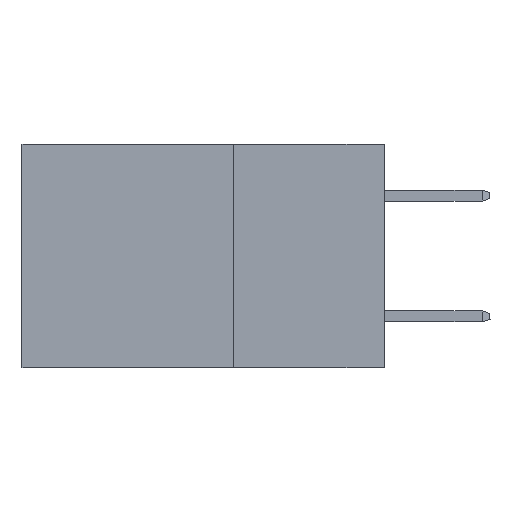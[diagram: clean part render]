
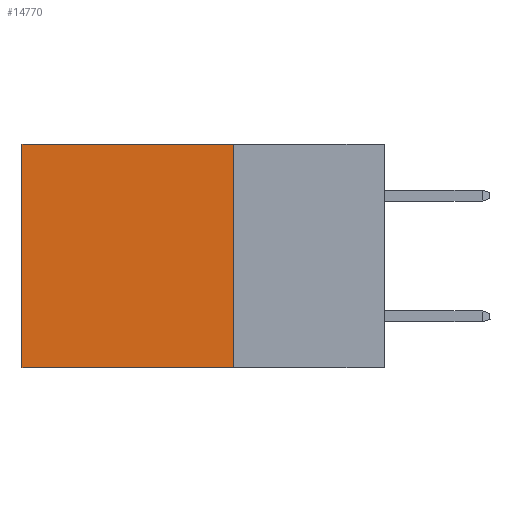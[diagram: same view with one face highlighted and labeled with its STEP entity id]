
A CAD part, left-side view. The second image highlights one B-rep face of the part: STEP entity #14770.
In plain terms, the highlighted planar face has unit normal (-1, 0, 0).
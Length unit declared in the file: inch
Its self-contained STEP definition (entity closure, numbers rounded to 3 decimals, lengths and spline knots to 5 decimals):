
#502 = CARTESIAN_POINT ( 'NONE',  ( 0.2615, 0.25, 0. ) ) ;
#1231 = ORIENTED_EDGE ( 'NONE', *, *, #18965, .T. ) ;
#3579 = EDGE_CURVE ( 'NONE', #19767, #16355, #6559, .T. ) ;
#3671 = DIRECTION ( 'NONE',  ( 0., 1., 0. ) ) ;
#4779 = VECTOR ( 'NONE', #6517, 39.37008 ) ;
#4913 = CARTESIAN_POINT ( 'NONE',  ( 0.2615, 0.25, -0.37 ) ) ;
#4959 = EDGE_CURVE ( 'NONE', #5180, #19767, #13064, .T. ) ;
#5180 = VERTEX_POINT ( 'NONE', #5378 ) ;
#5378 = CARTESIAN_POINT ( 'NONE',  ( 0.2615, 0.25, 0. ) ) ;
#5915 = CARTESIAN_POINT ( 'NONE',  ( 0.2615, 0.25, -0.37 ) ) ;
#5941 = LINE ( 'NONE', #502, #9126 ) ;
#6517 = DIRECTION ( 'NONE',  ( 0., 0., -1. ) ) ;
#6559 = LINE ( 'NONE', #12839, #9701 ) ;
#6846 = CARTESIAN_POINT ( 'NONE',  ( 0.2615, 0.6, -0.37 ) ) ;
#6908 = PLANE ( 'NONE',  #18008 ) ;
#8176 = CARTESIAN_POINT ( 'NONE',  ( 0.2615, 0.6, 0. ) ) ;
#8489 = DIRECTION ( 'NONE',  ( 0., 0., -1. ) ) ;
#9126 = VECTOR ( 'NONE', #3671, 39.37008 ) ;
#9701 = VECTOR ( 'NONE', #13713, 39.37008 ) ;
#11327 = EDGE_CURVE ( 'NONE', #5180, #20060, #5941, .T. ) ;
#11813 = EDGE_LOOP ( 'NONE', ( #1231, #12100, #13109, #17825 ) ) ;
#12100 = ORIENTED_EDGE ( 'NONE', *, *, #3579, .F. ) ;
#12839 = CARTESIAN_POINT ( 'NONE',  ( 0.2615, 0.25, -0.37 ) ) ;
#13064 = LINE ( 'NONE', #4913, #4779 ) ;
#13109 = ORIENTED_EDGE ( 'NONE', *, *, #4959, .F. ) ;
#13417 = CARTESIAN_POINT ( 'NONE',  ( 0.2615, 0.6, -0.37 ) ) ;
#13713 = DIRECTION ( 'NONE',  ( 0., 1., 0. ) ) ;
#14018 = VECTOR ( 'NONE', #18018, 39.37008 ) ;
#14601 = CARTESIAN_POINT ( 'NONE',  ( 0.2615, 0.25, -0.37 ) ) ;
#14770 = ADVANCED_FACE ( 'NONE', ( #18026 ), #6908, .F. ) ;
#16355 = VERTEX_POINT ( 'NONE', #6846 ) ;
#17676 = DIRECTION ( 'NONE',  ( 1., 0., 0. ) ) ;
#17825 = ORIENTED_EDGE ( 'NONE', *, *, #11327, .T. ) ;
#18008 = AXIS2_PLACEMENT_3D ( 'NONE', #14601, #17676, #8489 ) ;
#18018 = DIRECTION ( 'NONE',  ( 0., 0., -1. ) ) ;
#18026 = FACE_OUTER_BOUND ( 'NONE', #11813, .T. ) ;
#18098 = LINE ( 'NONE', #13417, #14018 ) ;
#18965 = EDGE_CURVE ( 'NONE', #20060, #16355, #18098, .T. ) ;
#19767 = VERTEX_POINT ( 'NONE', #5915 ) ;
#20060 = VERTEX_POINT ( 'NONE', #8176 ) ;
